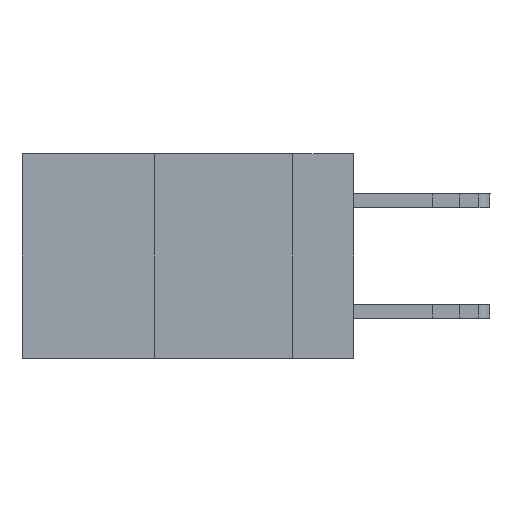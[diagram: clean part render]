
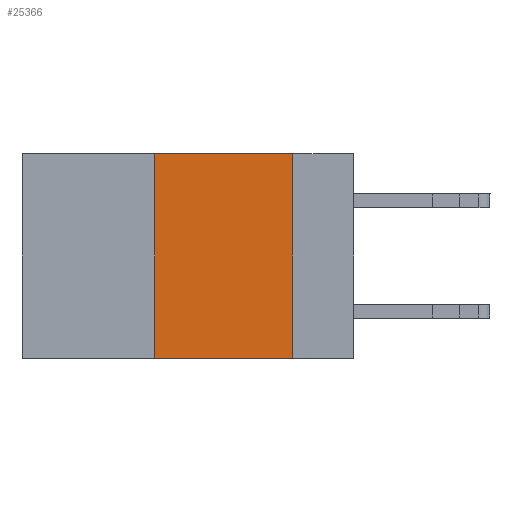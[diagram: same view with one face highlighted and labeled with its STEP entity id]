
A CAD part, left-side view. The second image highlights one B-rep face of the part: STEP entity #25366.
In plain terms, the highlighted planar face has unit normal (-1, 0, 0).
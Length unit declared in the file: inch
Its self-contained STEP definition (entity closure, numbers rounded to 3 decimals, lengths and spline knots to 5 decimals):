
#828 = CARTESIAN_POINT ( 'NONE',  ( 0., 0.6, -0.37 ) ) ;
#1817 = VERTEX_POINT ( 'NONE', #13031 ) ;
#2100 = EDGE_LOOP ( 'NONE', ( #12674, #13804, #22186, #14230 ) ) ;
#2646 = CARTESIAN_POINT ( 'NONE',  ( 0., 0.11, 0. ) ) ;
#3735 = VECTOR ( 'NONE', #5252, 39.37008 ) ;
#4887 = LINE ( 'NONE', #828, #21539 ) ;
#5252 = DIRECTION ( 'NONE',  ( 0., -1., 0. ) ) ;
#5889 = DIRECTION ( 'NONE',  ( 0., 0., -1. ) ) ;
#6177 = EDGE_CURVE ( 'NONE', #25040, #1817, #16394, .T. ) ;
#6459 = DIRECTION ( 'NONE',  ( 0., 0., -1. ) ) ;
#7337 = CARTESIAN_POINT ( 'NONE',  ( 0., 0.6, 0. ) ) ;
#8774 = VERTEX_POINT ( 'NONE', #11898 ) ;
#9679 = PLANE ( 'NONE',  #16564 ) ;
#10143 = EDGE_CURVE ( 'NONE', #8774, #14411, #16341, .T. ) ;
#11870 = FACE_OUTER_BOUND ( 'NONE', #2100, .T. ) ;
#11898 = CARTESIAN_POINT ( 'NONE',  ( 0., 0.36, -0.37 ) ) ;
#12674 = ORIENTED_EDGE ( 'NONE', *, *, #6177, .F. ) ;
#13031 = CARTESIAN_POINT ( 'NONE',  ( 0., 0.11, -0.37 ) ) ;
#13804 = ORIENTED_EDGE ( 'NONE', *, *, #14287, .F. ) ;
#14230 = ORIENTED_EDGE ( 'NONE', *, *, #23346, .T. ) ;
#14287 = EDGE_CURVE ( 'NONE', #14411, #25040, #15201, .T. ) ;
#14411 = VERTEX_POINT ( 'NONE', #23682 ) ;
#15201 = LINE ( 'NONE', #23561, #3735 ) ;
#16341 = LINE ( 'NONE', #24326, #18814 ) ;
#16394 = LINE ( 'NONE', #2646, #24228 ) ;
#16564 = AXIS2_PLACEMENT_3D ( 'NONE', #7337, #21448, #5889 ) ;
#18814 = VECTOR ( 'NONE', #22326, 39.37008 ) ;
#20977 = DIRECTION ( 'NONE',  ( 0., -1., 0. ) ) ;
#21448 = DIRECTION ( 'NONE',  ( 1., 0., 0. ) ) ;
#21539 = VECTOR ( 'NONE', #20977, 39.37008 ) ;
#22186 = ORIENTED_EDGE ( 'NONE', *, *, #10143, .F. ) ;
#22252 = CARTESIAN_POINT ( 'NONE',  ( 0., 0.11, 0. ) ) ;
#22326 = DIRECTION ( 'NONE',  ( 0., 0., 1. ) ) ;
#23346 = EDGE_CURVE ( 'NONE', #8774, #1817, #4887, .T. ) ;
#23561 = CARTESIAN_POINT ( 'NONE',  ( 0., 0.6, 0. ) ) ;
#23682 = CARTESIAN_POINT ( 'NONE',  ( 0., 0.36, 0. ) ) ;
#24228 = VECTOR ( 'NONE', #6459, 39.37008 ) ;
#24326 = CARTESIAN_POINT ( 'NONE',  ( 0., 0.36, 0. ) ) ;
#25040 = VERTEX_POINT ( 'NONE', #22252 ) ;
#25366 = ADVANCED_FACE ( 'NONE', ( #11870 ), #9679, .F. ) ;
